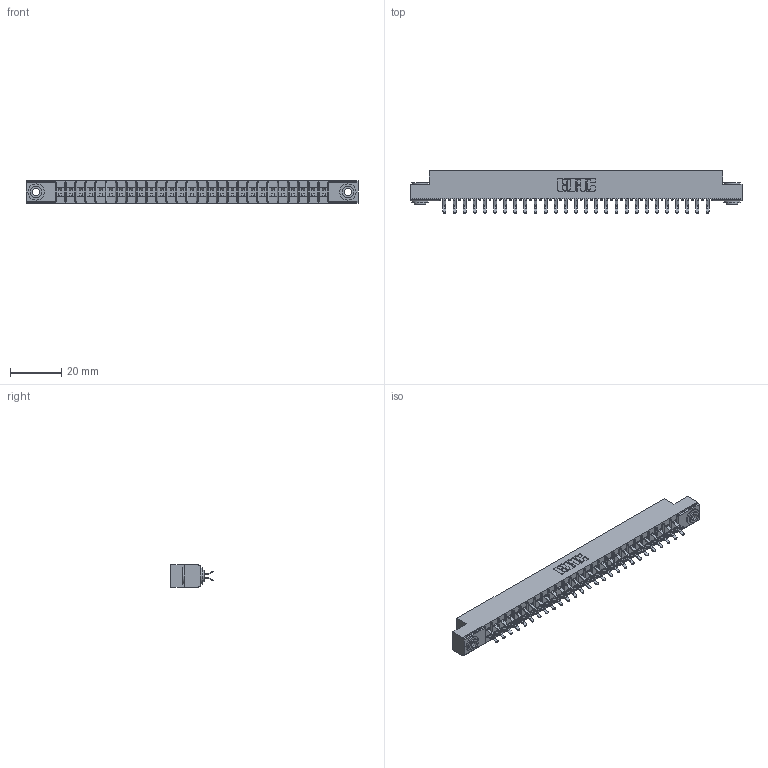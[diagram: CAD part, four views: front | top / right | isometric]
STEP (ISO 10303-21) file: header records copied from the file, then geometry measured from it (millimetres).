
FILE_DESCRIPTION (( 'STEP AP203' ), '1' );
FILE_NAME ('355-054-556-203.STEP', '2019-09-11T17:18:41', ( '' ), ( '' ), 'SwSTEP 2.0', 'SolidWorks 2016', '' );
FILE_SCHEMA (( 'CONFIG_CONTROL_DESIGN' ));
Length unit declared in the file: inch
Products named in the file (4): 305-290-001_556; 345-250-002_345-250-002-102; 305 Part_.156 Dia; 355-054-556-203
Assembly tree (57 placements, depth 2):
  355-054-556-203
    305 Part_.156 Dia
    305-290-001_556  x54
    345-250-002_345-250-002-102  x2
Bounding box: 130 x 16.64 x 8.71 mm (x, y, z)
Volume: 8134.5 mm3; surface area: 15933 mm2
Topology: 57 solids, 57 shells, 3192 faces, 9149 edges, 5950 vertices
Faces by surface type: plane 1766, cylinder 1310, sphere 108, cone 8
Entity records: 32347 total; most frequent: CARTESIAN_POINT 5336, ORIENTED_EDGE 5286, DIRECTION 5193, EDGE_CURVE 2643, VECTOR 2107, LINE 2107, VERTEX_POINT 1686, AXIS2_PLACEMENT_3D 1543
